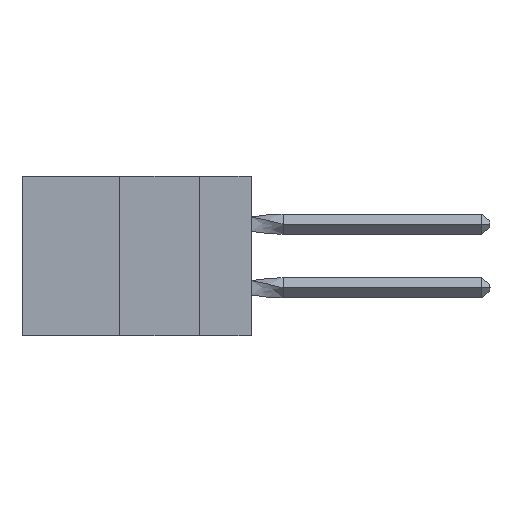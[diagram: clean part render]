
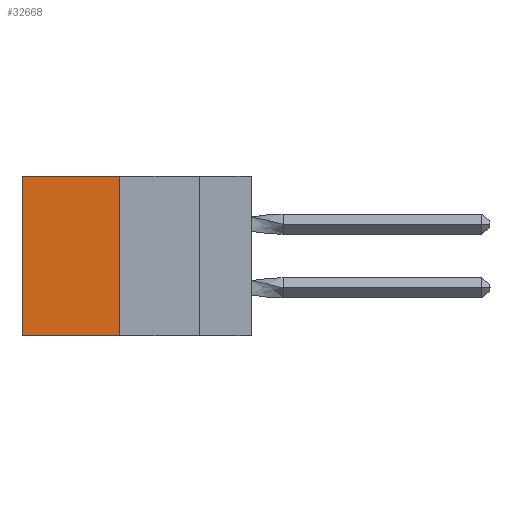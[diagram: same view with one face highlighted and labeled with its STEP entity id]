
A CAD part, left-side view. The second image highlights one B-rep face of the part: STEP entity #32668.
In plain terms, the highlighted planar face has unit normal (-1, 0, 0).
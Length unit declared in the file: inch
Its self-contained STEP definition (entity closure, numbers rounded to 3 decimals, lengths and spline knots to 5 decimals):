
#1235 = FACE_OUTER_BOUND ( 'NONE', #33107, .T. ) ;
#2185 = CARTESIAN_POINT ( 'NONE',  ( 0.305, 0.413, 0. ) ) ;
#2845 = ORIENTED_EDGE ( 'NONE', *, *, #12423, .T. ) ;
#3344 = ORIENTED_EDGE ( 'NONE', *, *, #23004, .F. ) ;
#5435 = CARTESIAN_POINT ( 'NONE',  ( 0.305, 0.72, -0.5 ) ) ;
#6682 = CARTESIAN_POINT ( 'NONE',  ( 0.305, 0.72, -0.5 ) ) ;
#8043 = DIRECTION ( 'NONE',  ( 0., 0., -1. ) ) ;
#8406 = LINE ( 'NONE', #5435, #28860 ) ;
#9101 = AXIS2_PLACEMENT_3D ( 'NONE', #29464, #23857, #24089 ) ;
#9593 = DIRECTION ( 'NONE',  ( 0., 1., 0. ) ) ;
#10523 = CARTESIAN_POINT ( 'NONE',  ( 0.305, 0.413, 0. ) ) ;
#10851 = VERTEX_POINT ( 'NONE', #10523 ) ;
#11014 = ORIENTED_EDGE ( 'NONE', *, *, #30568, .F. ) ;
#11573 = VECTOR ( 'NONE', #8043, 39.37008 ) ;
#12423 = EDGE_CURVE ( 'NONE', #26932, #24413, #8406, .T. ) ;
#12601 = LINE ( 'NONE', #17764, #30588 ) ;
#13225 = PLANE ( 'NONE',  #9101 ) ;
#15896 = EDGE_CURVE ( 'NONE', #10851, #26932, #32857, .T. ) ;
#17764 = CARTESIAN_POINT ( 'NONE',  ( 0.305, 0.413, -0.5 ) ) ;
#19996 = VERTEX_POINT ( 'NONE', #32215 ) ;
#22459 = LINE ( 'NONE', #23915, #11573 ) ;
#23004 = EDGE_CURVE ( 'NONE', #19996, #24413, #12601, .T. ) ;
#23857 = DIRECTION ( 'NONE',  ( 1., 0., 0. ) ) ;
#23915 = CARTESIAN_POINT ( 'NONE',  ( 0.305, 0.413, -0.5 ) ) ;
#24089 = DIRECTION ( 'NONE',  ( 0., 0., -1. ) ) ;
#24413 = VERTEX_POINT ( 'NONE', #6682 ) ;
#24829 = VECTOR ( 'NONE', #29233, 39.37008 ) ;
#25825 = CARTESIAN_POINT ( 'NONE',  ( 0.305, 0.72, 0. ) ) ;
#26932 = VERTEX_POINT ( 'NONE', #25825 ) ;
#28860 = VECTOR ( 'NONE', #32323, 39.37008 ) ;
#29233 = DIRECTION ( 'NONE',  ( 0., 1., 0. ) ) ;
#29464 = CARTESIAN_POINT ( 'NONE',  ( 0.305, 0.413, -0.5 ) ) ;
#30568 = EDGE_CURVE ( 'NONE', #10851, #19996, #22459, .T. ) ;
#30588 = VECTOR ( 'NONE', #9593, 39.37008 ) ;
#31084 = ORIENTED_EDGE ( 'NONE', *, *, #15896, .T. ) ;
#32215 = CARTESIAN_POINT ( 'NONE',  ( 0.305, 0.413, -0.5 ) ) ;
#32323 = DIRECTION ( 'NONE',  ( 0., 0., -1. ) ) ;
#32668 = ADVANCED_FACE ( 'NONE', ( #1235 ), #13225, .F. ) ;
#32857 = LINE ( 'NONE', #2185, #24829 ) ;
#33107 = EDGE_LOOP ( 'NONE', ( #2845, #3344, #11014, #31084 ) ) ;
